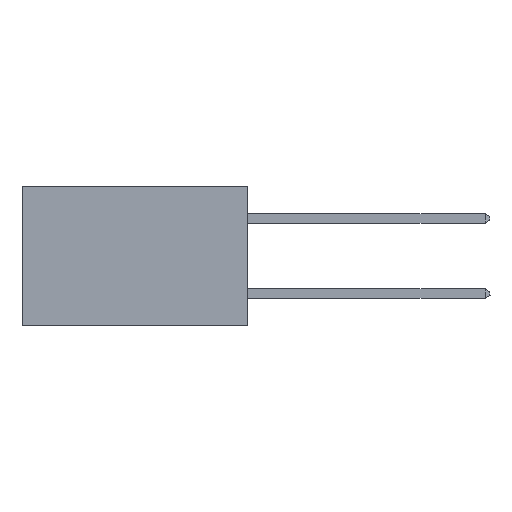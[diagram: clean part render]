
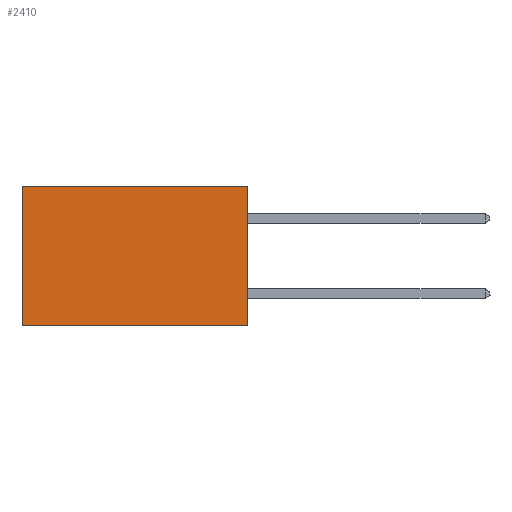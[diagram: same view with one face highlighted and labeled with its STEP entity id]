
A CAD part, left-side view. The second image highlights one B-rep face of the part: STEP entity #2410.
In plain terms, the highlighted planar face has unit normal (-1, 0, 0).
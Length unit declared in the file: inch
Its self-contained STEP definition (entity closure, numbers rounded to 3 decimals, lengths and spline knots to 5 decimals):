
#1943 = CARTESIAN_POINT ( 'NONE',  ( 0.298, 0., 0. ) ) ;
#2388 = CARTESIAN_POINT ( 'NONE',  ( 0.298, 0., 0. ) ) ;
#2410 = ADVANCED_FACE ( 'NONE', ( #17089 ), #26115, .F. ) ;
#3039 = LINE ( 'NONE', #10951, #16436 ) ;
#3595 = CARTESIAN_POINT ( 'NONE',  ( 0.298, 0., 0. ) ) ;
#4307 = ORIENTED_EDGE ( 'NONE', *, *, #24138, .T. ) ;
#6643 = DIRECTION ( 'NONE',  ( 0., 0., -1. ) ) ;
#8203 = DIRECTION ( 'NONE',  ( 0., 1., 0. ) ) ;
#8593 = EDGE_CURVE ( 'NONE', #14435, #15765, #3039, .T. ) ;
#9610 = LINE ( 'NONE', #1943, #14965 ) ;
#10951 = CARTESIAN_POINT ( 'NONE',  ( 0.298, 0., 0. ) ) ;
#11211 = ORIENTED_EDGE ( 'NONE', *, *, #22208, .F. ) ;
#11820 = ORIENTED_EDGE ( 'NONE', *, *, #8593, .F. ) ;
#13267 = DIRECTION ( 'NONE',  ( 0., 0., -1. ) ) ;
#14236 = DIRECTION ( 'NONE',  ( 0., 1., 0. ) ) ;
#14435 = VERTEX_POINT ( 'NONE', #3595 ) ;
#14965 = VECTOR ( 'NONE', #8203, 39.37008 ) ;
#15765 = VERTEX_POINT ( 'NONE', #27285 ) ;
#16436 = VECTOR ( 'NONE', #6643, 39.37008 ) ;
#17089 = FACE_OUTER_BOUND ( 'NONE', #22618, .T. ) ;
#17934 = VERTEX_POINT ( 'NONE', #21786 ) ;
#18606 = ORIENTED_EDGE ( 'NONE', *, *, #18986, .T. ) ;
#18857 = VECTOR ( 'NONE', #14236, 39.37008 ) ;
#18986 = EDGE_CURVE ( 'NONE', #14435, #23780, #9610, .T. ) ;
#19305 = CARTESIAN_POINT ( 'NONE',  ( 0.298, 0., -0.37 ) ) ;
#20414 = CARTESIAN_POINT ( 'NONE',  ( 0.298, 0.6, 0. ) ) ;
#21786 = CARTESIAN_POINT ( 'NONE',  ( 0.298, 0.6, -0.37 ) ) ;
#21992 = DIRECTION ( 'NONE',  ( 0., 0., -1. ) ) ;
#22208 = EDGE_CURVE ( 'NONE', #15765, #17934, #27574, .T. ) ;
#22346 = AXIS2_PLACEMENT_3D ( 'NONE', #2388, #24225, #21992 ) ;
#22434 = VECTOR ( 'NONE', #13267, 39.37008 ) ;
#22618 = EDGE_LOOP ( 'NONE', ( #4307, #11211, #11820, #18606 ) ) ;
#23780 = VERTEX_POINT ( 'NONE', #20414 ) ;
#23790 = LINE ( 'NONE', #23969, #22434 ) ;
#23969 = CARTESIAN_POINT ( 'NONE',  ( 0.298, 0.6, 0. ) ) ;
#24138 = EDGE_CURVE ( 'NONE', #23780, #17934, #23790, .T. ) ;
#24225 = DIRECTION ( 'NONE',  ( 1., 0., 0. ) ) ;
#26115 = PLANE ( 'NONE',  #22346 ) ;
#27285 = CARTESIAN_POINT ( 'NONE',  ( 0.298, 0., -0.37 ) ) ;
#27574 = LINE ( 'NONE', #19305, #18857 ) ;
